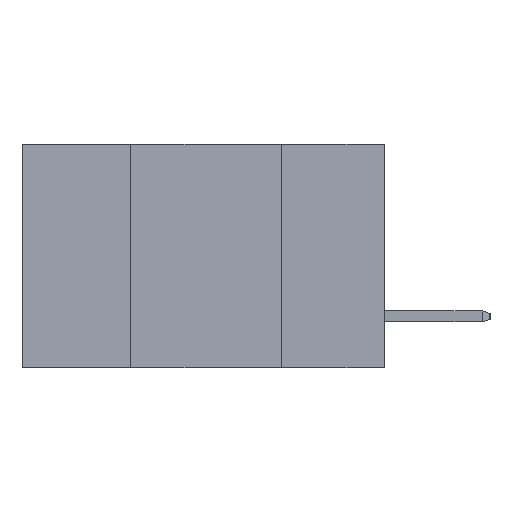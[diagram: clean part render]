
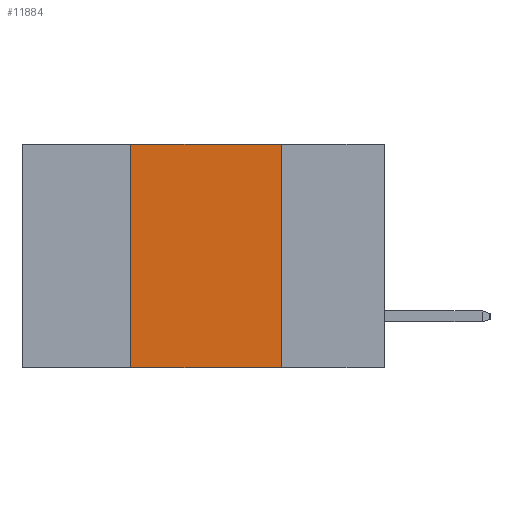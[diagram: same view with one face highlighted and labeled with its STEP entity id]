
A CAD part, left-side view. The second image highlights one B-rep face of the part: STEP entity #11884.
In plain terms, the highlighted planar face has unit normal (-1, 0, 0).
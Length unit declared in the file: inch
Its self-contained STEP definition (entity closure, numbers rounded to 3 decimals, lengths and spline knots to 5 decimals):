
#333 = LINE ( 'NONE', #13726, #4708 ) ;
#1300 = ORIENTED_EDGE ( 'NONE', *, *, #16186, .F. ) ;
#1514 = CARTESIAN_POINT ( 'NONE',  ( 0., 0.42, 0. ) ) ;
#1986 = AXIS2_PLACEMENT_3D ( 'NONE', #11102, #13652, #5851 ) ;
#2192 = ORIENTED_EDGE ( 'NONE', *, *, #3855, .F. ) ;
#2891 = VERTEX_POINT ( 'NONE', #9883 ) ;
#3036 = CARTESIAN_POINT ( 'NONE',  ( 0., 0.6, -0.37 ) ) ;
#3855 = EDGE_CURVE ( 'NONE', #5198, #6030, #16402, .T. ) ;
#4472 = PLANE ( 'NONE',  #1986 ) ;
#4708 = VECTOR ( 'NONE', #8659, 39.37008 ) ;
#5198 = VERTEX_POINT ( 'NONE', #1514 ) ;
#5602 = VECTOR ( 'NONE', #12396, 39.37008 ) ;
#5797 = VECTOR ( 'NONE', #10754, 39.37008 ) ;
#5851 = DIRECTION ( 'NONE',  ( 0., 0., -1. ) ) ;
#6030 = VERTEX_POINT ( 'NONE', #8755 ) ;
#8620 = EDGE_LOOP ( 'NONE', ( #11157, #2192, #1300, #15700 ) ) ;
#8659 = DIRECTION ( 'NONE',  ( 0., 0., -1. ) ) ;
#8755 = CARTESIAN_POINT ( 'NONE',  ( 0., 0.17, 0. ) ) ;
#8951 = FACE_OUTER_BOUND ( 'NONE', #8620, .T. ) ;
#9883 = CARTESIAN_POINT ( 'NONE',  ( 0., 0.42, -0.37 ) ) ;
#10754 = DIRECTION ( 'NONE',  ( 0., 0., 1. ) ) ;
#11102 = CARTESIAN_POINT ( 'NONE',  ( 0., 0.6, 0. ) ) ;
#11157 = ORIENTED_EDGE ( 'NONE', *, *, #17017, .F. ) ;
#11884 = ADVANCED_FACE ( 'NONE', ( #8951 ), #4472, .F. ) ;
#12396 = DIRECTION ( 'NONE',  ( 0., -1., 0. ) ) ;
#12601 = LINE ( 'NONE', #3036, #5602 ) ;
#12725 = VECTOR ( 'NONE', #15963, 39.37008 ) ;
#12764 = LINE ( 'NONE', #14500, #5797 ) ;
#13652 = DIRECTION ( 'NONE',  ( 1., 0., 0. ) ) ;
#13726 = CARTESIAN_POINT ( 'NONE',  ( 0., 0.17, 0. ) ) ;
#14500 = CARTESIAN_POINT ( 'NONE',  ( 0., 0.42, 0. ) ) ;
#14697 = CARTESIAN_POINT ( 'NONE',  ( 0., 0.6, 0. ) ) ;
#15367 = EDGE_CURVE ( 'NONE', #2891, #16214, #12601, .T. ) ;
#15700 = ORIENTED_EDGE ( 'NONE', *, *, #15367, .T. ) ;
#15963 = DIRECTION ( 'NONE',  ( 0., -1., 0. ) ) ;
#16186 = EDGE_CURVE ( 'NONE', #2891, #5198, #12764, .T. ) ;
#16214 = VERTEX_POINT ( 'NONE', #17047 ) ;
#16402 = LINE ( 'NONE', #14697, #12725 ) ;
#17017 = EDGE_CURVE ( 'NONE', #6030, #16214, #333, .T. ) ;
#17047 = CARTESIAN_POINT ( 'NONE',  ( 0., 0.17, -0.37 ) ) ;
